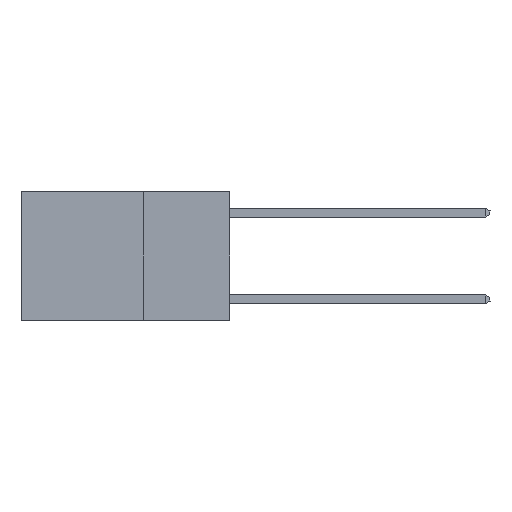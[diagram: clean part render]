
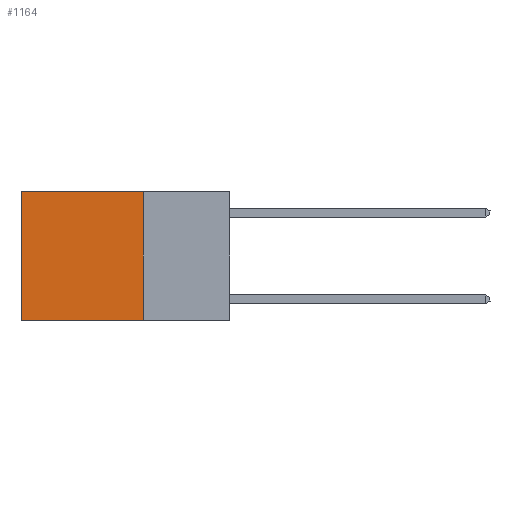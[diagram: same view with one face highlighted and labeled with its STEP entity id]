
A CAD part, left-side view. The second image highlights one B-rep face of the part: STEP entity #1164.
In plain terms, the highlighted planar face has unit normal (-1, 0, 0).
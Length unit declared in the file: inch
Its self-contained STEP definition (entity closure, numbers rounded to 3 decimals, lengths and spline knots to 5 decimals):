
#1164 = ADVANCED_FACE ( 'NONE', ( #7516 ), #11979, .F. ) ;
#1378 = CARTESIAN_POINT ( 'NONE',  ( 0.2625, 0.6, 0. ) ) ;
#1964 = VECTOR ( 'NONE', #15737, 39.37008 ) ;
#2387 = ORIENTED_EDGE ( 'NONE', *, *, #19400, .T. ) ;
#3186 = LINE ( 'NONE', #13361, #25152 ) ;
#3497 = CARTESIAN_POINT ( 'NONE',  ( 0.2625, 0.25, 0. ) ) ;
#4067 = CARTESIAN_POINT ( 'NONE',  ( 0.2625, 0.6, 0. ) ) ;
#5005 = CARTESIAN_POINT ( 'NONE',  ( 0.2625, 0.25, 0. ) ) ;
#6237 = VECTOR ( 'NONE', #11956, 39.37008 ) ;
#6246 = CARTESIAN_POINT ( 'NONE',  ( 0.2625, 0.25, -0.37 ) ) ;
#7516 = FACE_OUTER_BOUND ( 'NONE', #22098, .T. ) ;
#9681 = VERTEX_POINT ( 'NONE', #6246 ) ;
#9879 = DIRECTION ( 'NONE',  ( 1., 0., 0. ) ) ;
#11071 = VECTOR ( 'NONE', #14740, 39.37008 ) ;
#11176 = EDGE_CURVE ( 'NONE', #12448, #9681, #21130, .T. ) ;
#11530 = DIRECTION ( 'NONE',  ( 0., 1., 0. ) ) ;
#11699 = CARTESIAN_POINT ( 'NONE',  ( 0.2625, 0.25, 0. ) ) ;
#11956 = DIRECTION ( 'NONE',  ( 0., 0., -1. ) ) ;
#11979 = PLANE ( 'NONE',  #15788 ) ;
#12448 = VERTEX_POINT ( 'NONE', #5005 ) ;
#12671 = EDGE_CURVE ( 'NONE', #20708, #27098, #24470, .T. ) ;
#12846 = ORIENTED_EDGE ( 'NONE', *, *, #11176, .F. ) ;
#13361 = CARTESIAN_POINT ( 'NONE',  ( 0.2625, 0.25, -0.37 ) ) ;
#14740 = DIRECTION ( 'NONE',  ( 0., 0., -1. ) ) ;
#15737 = DIRECTION ( 'NONE',  ( 0., 1., 0. ) ) ;
#15782 = ORIENTED_EDGE ( 'NONE', *, *, #12671, .T. ) ;
#15788 = AXIS2_PLACEMENT_3D ( 'NONE', #11699, #9879, #20464 ) ;
#18897 = CARTESIAN_POINT ( 'NONE',  ( 0.2625, 0.25, 0. ) ) ;
#19400 = EDGE_CURVE ( 'NONE', #12448, #20708, #24638, .T. ) ;
#20464 = DIRECTION ( 'NONE',  ( 0., 0., -1. ) ) ;
#20570 = CARTESIAN_POINT ( 'NONE',  ( 0.2625, 0.6, -0.37 ) ) ;
#20708 = VERTEX_POINT ( 'NONE', #4067 ) ;
#21130 = LINE ( 'NONE', #18897, #11071 ) ;
#22098 = EDGE_LOOP ( 'NONE', ( #15782, #22438, #12846, #2387 ) ) ;
#22438 = ORIENTED_EDGE ( 'NONE', *, *, #24073, .F. ) ;
#24073 = EDGE_CURVE ( 'NONE', #9681, #27098, #3186, .T. ) ;
#24470 = LINE ( 'NONE', #1378, #6237 ) ;
#24638 = LINE ( 'NONE', #3497, #1964 ) ;
#25152 = VECTOR ( 'NONE', #11530, 39.37008 ) ;
#27098 = VERTEX_POINT ( 'NONE', #20570 ) ;
